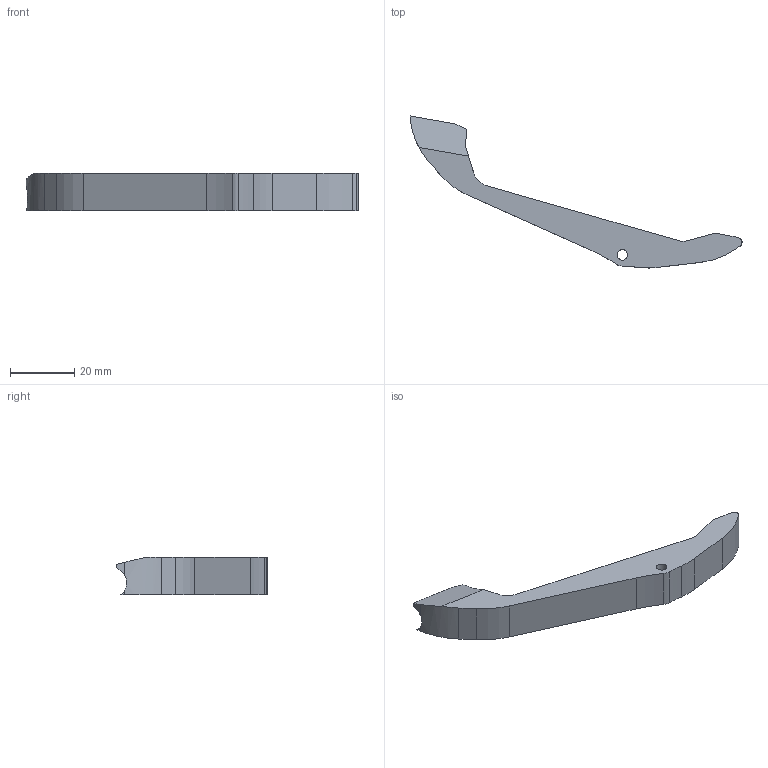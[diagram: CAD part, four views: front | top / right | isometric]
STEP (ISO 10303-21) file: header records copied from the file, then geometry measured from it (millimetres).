
FILE_DESCRIPTION(/* description */ (''),/* implementation_level */ '2;1');
FILE_NAME(/* name */ 'Ejector.step',/* time_stamp */ '2022-05-11T21:19:23-06:00',/* author */ (''),/* organization */ (''),/* preprocessor_version */ 'ST-DEVELOPER v18.1',/* originating_system */ 'Autodesk Translation Framework v10.10.0.1391',/* authorisation */ '');
FILE_SCHEMA (('AUTOMOTIVE_DESIGN { 1 0 10303 214 3 1 1 }'));
Length unit declared in the file: millimetre
Products named in the file (1): Ejector
Bounding box: 103.66 x 47.45 x 11.85 mm (x, y, z)
Volume: 11416.3 mm3; surface area: 4966 mm2
Topology: 1 solids, 1 shells, 32 faces, 89 edges, 59 vertices
Faces by surface type: cylinder 16, plane 15, bspline 1
Full cylindrical faces by diameter (mm): 3.25 x1
Entity records: 1148 total; most frequent: CARTESIAN_POINT 267, ORIENTED_EDGE 178, DIRECTION 176, EDGE_CURVE 89, AXIS2_PLACEMENT_3D 62, VERTEX_POINT 59, LINE 52, VECTOR 52
